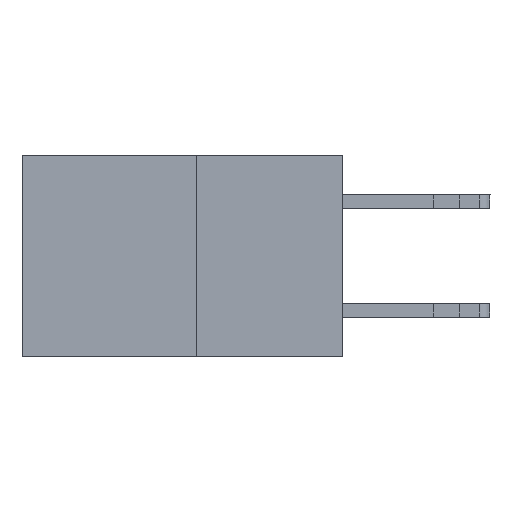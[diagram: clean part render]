
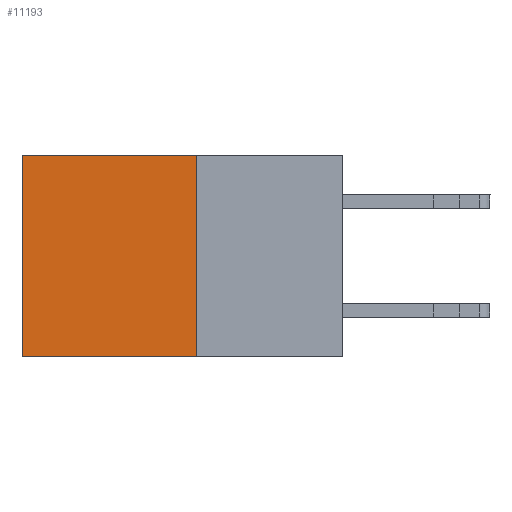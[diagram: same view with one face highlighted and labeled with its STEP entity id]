
A CAD part, left-side view. The second image highlights one B-rep face of the part: STEP entity #11193.
In plain terms, the highlighted planar face has unit normal (-1, 0, 0).
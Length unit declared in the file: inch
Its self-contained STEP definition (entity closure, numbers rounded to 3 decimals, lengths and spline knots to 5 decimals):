
#94 = LINE ( 'NONE', #9139, #3958 ) ;
#2851 = ORIENTED_EDGE ( 'NONE', *, *, #10976, .T. ) ;
#2879 = DIRECTION ( 'NONE',  ( 1., 0., 0. ) ) ;
#3664 = VECTOR ( 'NONE', #6504, 39.37008 ) ;
#3775 = VERTEX_POINT ( 'NONE', #17670 ) ;
#3958 = VECTOR ( 'NONE', #16832, 39.37008 ) ;
#4648 = ORIENTED_EDGE ( 'NONE', *, *, #11846, .F. ) ;
#6080 = PLANE ( 'NONE',  #7315 ) ;
#6504 = DIRECTION ( 'NONE',  ( 0., 1., 0. ) ) ;
#6753 = CARTESIAN_POINT ( 'NONE',  ( 0.277, 0.27, 0. ) ) ;
#7148 = VERTEX_POINT ( 'NONE', #11844 ) ;
#7228 = CARTESIAN_POINT ( 'NONE',  ( 0.277, 0.27, 0. ) ) ;
#7315 = AXIS2_PLACEMENT_3D ( 'NONE', #12385, #2879, #14007 ) ;
#8991 = CARTESIAN_POINT ( 'NONE',  ( 0.277, 0.59, -0.37 ) ) ;
#9139 = CARTESIAN_POINT ( 'NONE',  ( 0.277, 0.27, -0.37 ) ) ;
#9448 = VECTOR ( 'NONE', #19580, 39.37008 ) ;
#10015 = VERTEX_POINT ( 'NONE', #6753 ) ;
#10360 = EDGE_CURVE ( 'NONE', #15643, #3775, #13659, .T. ) ;
#10877 = FACE_OUTER_BOUND ( 'NONE', #16384, .T. ) ;
#10976 = EDGE_CURVE ( 'NONE', #10015, #15643, #11123, .T. ) ;
#11123 = LINE ( 'NONE', #7228, #15745 ) ;
#11193 = ADVANCED_FACE ( 'NONE', ( #10877 ), #6080, .F. ) ;
#11844 = CARTESIAN_POINT ( 'NONE',  ( 0.277, 0.27, -0.37 ) ) ;
#11846 = EDGE_CURVE ( 'NONE', #10015, #7148, #94, .T. ) ;
#12076 = LINE ( 'NONE', #18675, #3664 ) ;
#12385 = CARTESIAN_POINT ( 'NONE',  ( 0.277, 0.27, -0.37 ) ) ;
#13021 = ORIENTED_EDGE ( 'NONE', *, *, #18031, .F. ) ;
#13472 = DIRECTION ( 'NONE',  ( 0., 1., 0. ) ) ;
#13659 = LINE ( 'NONE', #8991, #9448 ) ;
#14007 = DIRECTION ( 'NONE',  ( 0., 0., -1. ) ) ;
#14745 = ORIENTED_EDGE ( 'NONE', *, *, #10360, .T. ) ;
#15643 = VERTEX_POINT ( 'NONE', #18373 ) ;
#15745 = VECTOR ( 'NONE', #13472, 39.37008 ) ;
#16384 = EDGE_LOOP ( 'NONE', ( #14745, #13021, #4648, #2851 ) ) ;
#16832 = DIRECTION ( 'NONE',  ( 0., 0., -1. ) ) ;
#17670 = CARTESIAN_POINT ( 'NONE',  ( 0.277, 0.59, -0.37 ) ) ;
#18031 = EDGE_CURVE ( 'NONE', #7148, #3775, #12076, .T. ) ;
#18373 = CARTESIAN_POINT ( 'NONE',  ( 0.277, 0.59, 0. ) ) ;
#18675 = CARTESIAN_POINT ( 'NONE',  ( 0.277, 0.27, -0.37 ) ) ;
#19580 = DIRECTION ( 'NONE',  ( 0., 0., -1. ) ) ;
